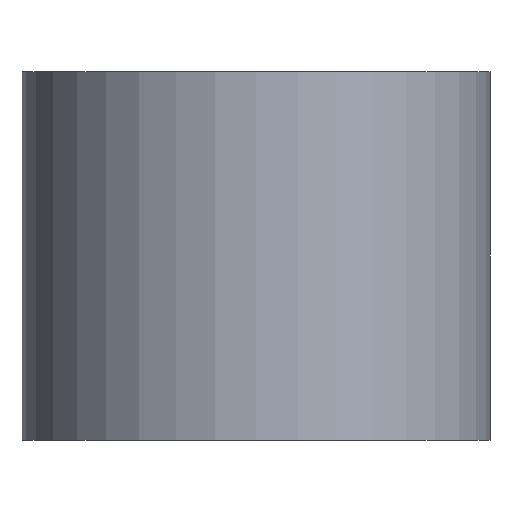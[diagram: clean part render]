
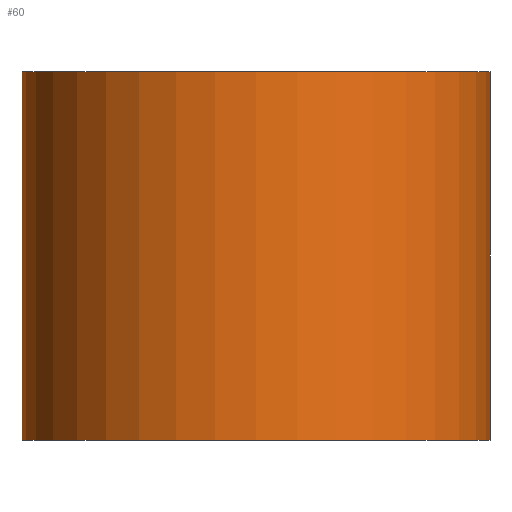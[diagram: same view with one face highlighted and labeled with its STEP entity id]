
A CAD part, front view. The second image highlights one B-rep face of the part: STEP entity #60.
In plain terms, the highlighted cylindrical face has radius 6.35 mm (diameter 12.7 mm), a full revolution.
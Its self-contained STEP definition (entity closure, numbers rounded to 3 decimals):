
#1 = CARTESIAN_POINT ( 'NONE',  ( 6.35, 0., 0. ) ) ;
#7 = FACE_OUTER_BOUND ( 'NONE', #44, .T. ) ;
#10 = CIRCLE ( 'NONE', #169, 6.35 ) ;
#26 = DIRECTION ( 'NONE',  ( 0., 0., 1. ) ) ;
#28 = EDGE_CURVE ( 'NONE', #139, #139, #49, .T. ) ;
#29 = CARTESIAN_POINT ( 'NONE',  ( 0., 0., 10. ) ) ;
#41 = DIRECTION ( 'NONE',  ( 1., 0., 0. ) ) ;
#44 = EDGE_LOOP ( 'NONE', ( #53 ) ) ;
#49 = CIRCLE ( 'NONE', #66, 6.35 ) ;
#53 = ORIENTED_EDGE ( 'NONE', *, *, #28, .F. ) ;
#60 = ADVANCED_FACE ( 'NONE', ( #7, #155 ), #112, .T. ) ;
#66 = AXIS2_PLACEMENT_3D ( 'NONE', #29, #26, #81 ) ;
#81 = DIRECTION ( 'NONE',  ( 1., 0., 0. ) ) ;
#97 = CARTESIAN_POINT ( 'NONE',  ( 0., 0., 0. ) ) ;
#100 = CARTESIAN_POINT ( 'NONE',  ( 0., 0., 0. ) ) ;
#107 = EDGE_LOOP ( 'NONE', ( #137 ) ) ;
#112 = CYLINDRICAL_SURFACE ( 'NONE', #161, 6.35 ) ;
#128 = VERTEX_POINT ( 'NONE', #1 ) ;
#130 = CARTESIAN_POINT ( 'NONE',  ( 6.35, 0., 10. ) ) ;
#133 = DIRECTION ( 'NONE',  ( 1., 0., 0. ) ) ;
#137 = ORIENTED_EDGE ( 'NONE', *, *, #167, .T. ) ;
#139 = VERTEX_POINT ( 'NONE', #130 ) ;
#155 = FACE_OUTER_BOUND ( 'NONE', #107, .T. ) ;
#157 = DIRECTION ( 'NONE',  ( 0., 0., 1. ) ) ;
#158 = DIRECTION ( 'NONE',  ( 0., 0., -1. ) ) ;
#161 = AXIS2_PLACEMENT_3D ( 'NONE', #100, #158, #133 ) ;
#167 = EDGE_CURVE ( 'NONE', #128, #128, #10, .T. ) ;
#169 = AXIS2_PLACEMENT_3D ( 'NONE', #97, #157, #41 ) ;
